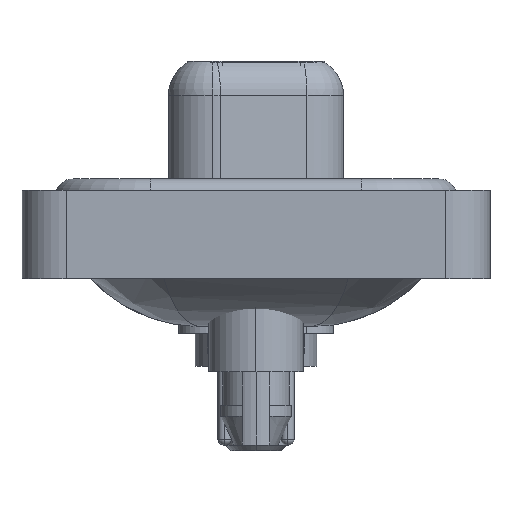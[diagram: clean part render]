
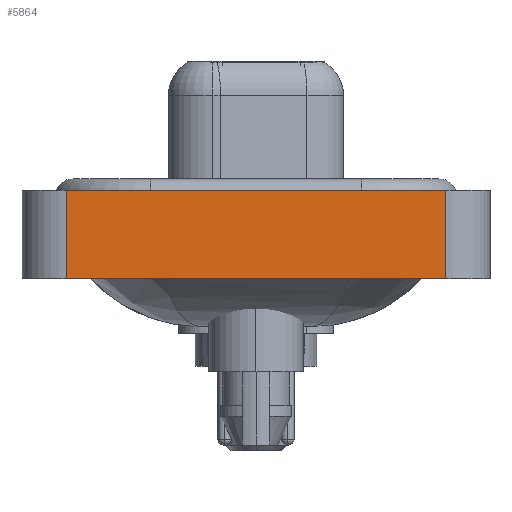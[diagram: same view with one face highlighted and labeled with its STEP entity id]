
A CAD part, left-side view. The second image highlights one B-rep face of the part: STEP entity #5864.
In plain terms, the highlighted planar face has unit normal (-1, 0, 0).
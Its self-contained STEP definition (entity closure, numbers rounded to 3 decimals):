
#231 = CARTESIAN_POINT ( 'NONE',  ( -7.25, 8.55, -3.6 ) ) ;
#337 = VECTOR ( 'NONE', #9981, 1000. ) ;
#702 = CARTESIAN_POINT ( 'NONE',  ( -7.25, -8.55, 0.4 ) ) ;
#744 = CARTESIAN_POINT ( 'NONE',  ( -7.25, -8.55, -3.6 ) ) ;
#2133 = VERTEX_POINT ( 'NONE', #10669 ) ;
#3225 = CARTESIAN_POINT ( 'NONE',  ( -7.25, 8.55, -3.6 ) ) ;
#3311 = EDGE_CURVE ( 'NONE', #18070, #9795, #3834, .T. ) ;
#3466 = LINE ( 'NONE', #744, #337 ) ;
#3834 = LINE ( 'NONE', #702, #11174 ) ;
#4083 = LINE ( 'NONE', #12146, #18656 ) ;
#5135 = DIRECTION ( 'NONE',  ( 0., 0., 1. ) ) ;
#5580 = DIRECTION ( 'NONE',  ( 0., -1., 0. ) ) ;
#5864 = ADVANCED_FACE ( 'NONE', ( #13314 ), #18206, .T. ) ;
#9795 = VERTEX_POINT ( 'NONE', #17325 ) ;
#9981 = DIRECTION ( 'NONE',  ( 0., 0., 1. ) ) ;
#10669 = CARTESIAN_POINT ( 'NONE',  ( -7.25, -8.55, -3.6 ) ) ;
#10687 = ORIENTED_EDGE ( 'NONE', *, *, #14155, .F. ) ;
#10997 = LINE ( 'NONE', #3225, #19910 ) ;
#11001 = ORIENTED_EDGE ( 'NONE', *, *, #3311, .F. ) ;
#11174 = VECTOR ( 'NONE', #5580, 1000. ) ;
#11823 = EDGE_CURVE ( 'NONE', #2133, #9795, #3466, .T. ) ;
#12146 = CARTESIAN_POINT ( 'NONE',  ( -7.25, -8.55, -3.6 ) ) ;
#12437 = DIRECTION ( 'NONE',  ( 0., 0., 1. ) ) ;
#12793 = ORIENTED_EDGE ( 'NONE', *, *, #11823, .T. ) ;
#13314 = FACE_OUTER_BOUND ( 'NONE', #19136, .T. ) ;
#13490 = ORIENTED_EDGE ( 'NONE', *, *, #19037, .T. ) ;
#14155 = EDGE_CURVE ( 'NONE', #15518, #18070, #10997, .T. ) ;
#14888 = DIRECTION ( 'NONE',  ( -1., 0., 0. ) ) ;
#15518 = VERTEX_POINT ( 'NONE', #231 ) ;
#16724 = AXIS2_PLACEMENT_3D ( 'NONE', #19749, #14888, #5135 ) ;
#17041 = CARTESIAN_POINT ( 'NONE',  ( -7.25, 8.55, 0.4 ) ) ;
#17325 = CARTESIAN_POINT ( 'NONE',  ( -7.25, -8.55, 0.4 ) ) ;
#18070 = VERTEX_POINT ( 'NONE', #17041 ) ;
#18206 = PLANE ( 'NONE',  #16724 ) ;
#18656 = VECTOR ( 'NONE', #20348, 1000. ) ;
#19037 = EDGE_CURVE ( 'NONE', #15518, #2133, #4083, .T. ) ;
#19136 = EDGE_LOOP ( 'NONE', ( #12793, #11001, #10687, #13490 ) ) ;
#19749 = CARTESIAN_POINT ( 'NONE',  ( -7.25, -8.55, -3.6 ) ) ;
#19910 = VECTOR ( 'NONE', #12437, 1000. ) ;
#20348 = DIRECTION ( 'NONE',  ( 0., -1., 0. ) ) ;
